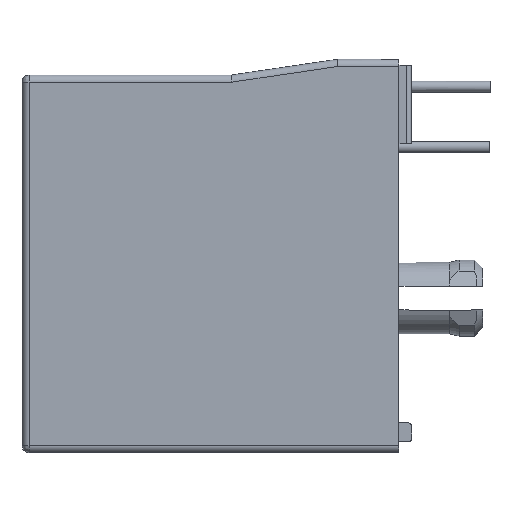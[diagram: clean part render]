
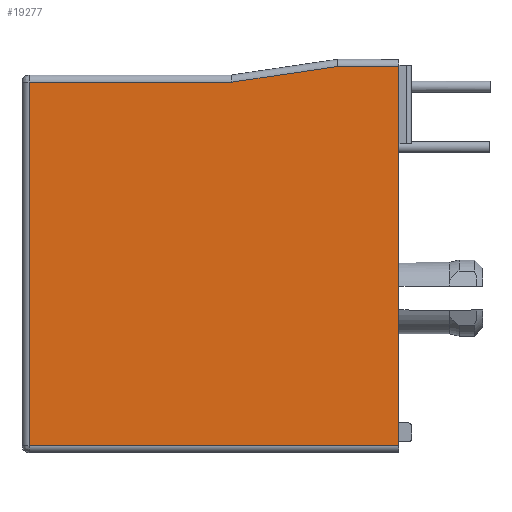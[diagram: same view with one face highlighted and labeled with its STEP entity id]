
A CAD part, left-side view. The second image highlights one B-rep face of the part: STEP entity #19277.
In plain terms, the highlighted planar face has unit normal (-1, 0, 0).
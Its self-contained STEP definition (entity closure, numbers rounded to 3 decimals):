
#115 = CARTESIAN_POINT ( 'NONE',  ( -7.68, 7.64, 9.08 ) ) ;
#246 = CARTESIAN_POINT ( 'NONE',  ( -7.68, -7.91, 9.74 ) ) ;
#1200 = DIRECTION ( 'NONE',  ( 0., 0., 1. ) ) ;
#1646 = CARTESIAN_POINT ( 'NONE',  ( -7.68, 7.64, 9.74 ) ) ;
#1810 = PLANE ( 'NONE',  #6068 ) ;
#2032 = VERTEX_POINT ( 'NONE', #115 ) ;
#2608 = CARTESIAN_POINT ( 'NONE',  ( -7.68, -5.332, 9.74 ) ) ;
#3064 = LINE ( 'NONE', #1646, #8669 ) ;
#3125 = DIRECTION ( 'NONE',  ( -1., 0., 0. ) ) ;
#3584 = DIRECTION ( 'NONE',  ( 0., -1., 0. ) ) ;
#3605 = LINE ( 'NONE', #10949, #14024 ) ;
#3745 = CARTESIAN_POINT ( 'NONE',  ( -7.68, -7.91, 9.74 ) ) ;
#4099 = VERTEX_POINT ( 'NONE', #8749 ) ;
#4183 = FACE_OUTER_BOUND ( 'NONE', #17072, .T. ) ;
#4558 = CARTESIAN_POINT ( 'NONE',  ( -7.68, -5.332, 9.74 ) ) ;
#4750 = EDGE_CURVE ( 'NONE', #14075, #4830, #11566, .T. ) ;
#4830 = VERTEX_POINT ( 'NONE', #6090 ) ;
#4917 = EDGE_CURVE ( 'NONE', #2032, #14075, #3064, .T. ) ;
#5042 = EDGE_CURVE ( 'NONE', #4099, #2032, #14455, .T. ) ;
#5211 = CARTESIAN_POINT ( 'NONE',  ( -7.68, -7.91, 9.08 ) ) ;
#5636 = ORIENTED_EDGE ( 'NONE', *, *, #8754, .T. ) ;
#5969 = DIRECTION ( 'NONE',  ( 0., 0.989, -0.147 ) ) ;
#6057 = VECTOR ( 'NONE', #5969, 1000. ) ;
#6068 = AXIS2_PLACEMENT_3D ( 'NONE', #246, #3125, #18741 ) ;
#6090 = CARTESIAN_POINT ( 'NONE',  ( -7.68, -7.91, -6.2 ) ) ;
#6255 = LINE ( 'NONE', #18141, #12087 ) ;
#7395 = VERTEX_POINT ( 'NONE', #2608 ) ;
#8034 = LINE ( 'NONE', #4558, #6057 ) ;
#8301 = CARTESIAN_POINT ( 'NONE',  ( -7.68, -7.91, -6.2 ) ) ;
#8461 = ORIENTED_EDGE ( 'NONE', *, *, #4750, .T. ) ;
#8593 = VERTEX_POINT ( 'NONE', #3745 ) ;
#8669 = VECTOR ( 'NONE', #15747, 1000. ) ;
#8709 = CARTESIAN_POINT ( 'NONE',  ( -7.68, 7.64, -6.2 ) ) ;
#8749 = CARTESIAN_POINT ( 'NONE',  ( -7.68, -0.882, 9.08 ) ) ;
#8754 = EDGE_CURVE ( 'NONE', #7395, #4099, #8034, .T. ) ;
#9606 = EDGE_CURVE ( 'NONE', #8593, #7395, #3605, .T. ) ;
#9946 = EDGE_CURVE ( 'NONE', #4830, #8593, #6255, .T. ) ;
#10676 = ORIENTED_EDGE ( 'NONE', *, *, #5042, .T. ) ;
#10949 = CARTESIAN_POINT ( 'NONE',  ( -7.68, -7.91, 9.74 ) ) ;
#11566 = LINE ( 'NONE', #8301, #19505 ) ;
#11850 = ORIENTED_EDGE ( 'NONE', *, *, #9946, .T. ) ;
#12087 = VECTOR ( 'NONE', #1200, 1000. ) ;
#13479 = VECTOR ( 'NONE', #16017, 1000. ) ;
#14024 = VECTOR ( 'NONE', #14060, 1000. ) ;
#14060 = DIRECTION ( 'NONE',  ( 0., 1., 0. ) ) ;
#14075 = VERTEX_POINT ( 'NONE', #8709 ) ;
#14455 = LINE ( 'NONE', #5211, #13479 ) ;
#15747 = DIRECTION ( 'NONE',  ( 0., 0., -1. ) ) ;
#16017 = DIRECTION ( 'NONE',  ( 0., 1., 0. ) ) ;
#16340 = ORIENTED_EDGE ( 'NONE', *, *, #9606, .T. ) ;
#17072 = EDGE_LOOP ( 'NONE', ( #5636, #10676, #19847, #8461, #11850, #16340 ) ) ;
#18141 = CARTESIAN_POINT ( 'NONE',  ( -7.68, -7.91, 9.74 ) ) ;
#18741 = DIRECTION ( 'NONE',  ( 0., 0., 1. ) ) ;
#19277 = ADVANCED_FACE ( 'NONE', ( #4183 ), #1810, .T. ) ;
#19505 = VECTOR ( 'NONE', #3584, 1000. ) ;
#19847 = ORIENTED_EDGE ( 'NONE', *, *, #4917, .T. ) ;
